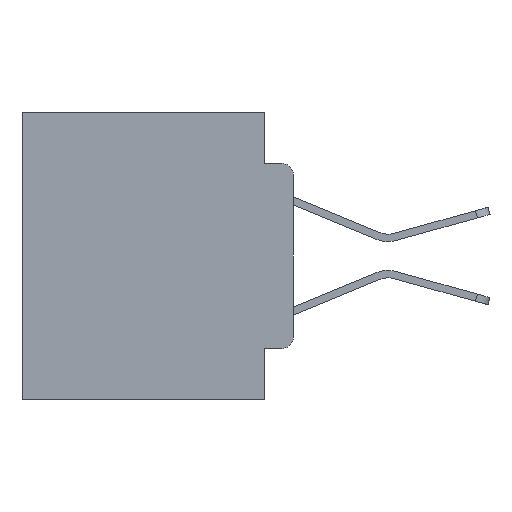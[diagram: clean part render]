
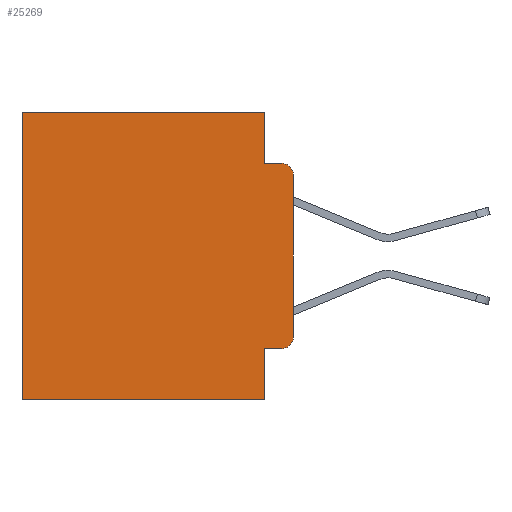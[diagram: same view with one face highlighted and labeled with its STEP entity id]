
A CAD part, left-side view. The second image highlights one B-rep face of the part: STEP entity #25269.
In plain terms, the highlighted planar face has unit normal (-1, 0, 0).
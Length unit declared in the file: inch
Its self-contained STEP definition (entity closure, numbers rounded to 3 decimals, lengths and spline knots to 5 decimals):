
#280 = ORIENTED_EDGE ( 'NONE', *, *, #2390, .T. ) ;
#667 = ORIENTED_EDGE ( 'NONE', *, *, #17414, .T. ) ;
#914 = FACE_OUTER_BOUND ( 'NONE', #7038, .T. ) ;
#1021 = ORIENTED_EDGE ( 'NONE', *, *, #18911, .T. ) ;
#1097 = ORIENTED_EDGE ( 'NONE', *, *, #22683, .F. ) ;
#1190 = CARTESIAN_POINT ( 'NONE',  ( 0.298, 0.051, -0.0885 ) ) ;
#1203 = DIRECTION ( 'NONE',  ( 0., 0., -1. ) ) ;
#1210 = EDGE_CURVE ( 'NONE', #7250, #12770, #22981, .T. ) ;
#1242 = ORIENTED_EDGE ( 'NONE', *, *, #22350, .F. ) ;
#1360 = LINE ( 'NONE', #16604, #23978 ) ;
#1700 = ORIENTED_EDGE ( 'NONE', *, *, #28054, .T. ) ;
#1843 = ORIENTED_EDGE ( 'NONE', *, *, #1210, .F. ) ;
#1898 = ORIENTED_EDGE ( 'NONE', *, *, #25222, .F. ) ;
#2041 = ORIENTED_EDGE ( 'NONE', *, *, #22127, .T. ) ;
#2135 = LINE ( 'NONE', #11034, #7387 ) ;
#2136 = ORIENTED_EDGE ( 'NONE', *, *, #23571, .F. ) ;
#2301 = CARTESIAN_POINT ( 'NONE',  ( 0.298, 0.051, -0.0885 ) ) ;
#2390 = EDGE_CURVE ( 'NONE', #7785, #23870, #25370, .T. ) ;
#3108 = LINE ( 'NONE', #10858, #14094 ) ;
#3114 = LINE ( 'NONE', #22416, #19875 ) ;
#3369 = CARTESIAN_POINT ( 'NONE',  ( 0.298, 0.051, 0. ) ) ;
#4490 = VERTEX_POINT ( 'NONE', #23769 ) ;
#4699 = CIRCLE ( 'NONE', #20246, 0.02 ) ;
#4994 = CARTESIAN_POINT ( 'NONE',  ( 0.298, 0., 0. ) ) ;
#5281 = DIRECTION ( 'NONE',  ( 0., -1., 0. ) ) ;
#5590 = DIRECTION ( 'NONE',  ( 0., 0., -1. ) ) ;
#6176 = LINE ( 'NONE', #26928, #27866 ) ;
#6746 = DIRECTION ( 'NONE',  ( 1., 0., 0. ) ) ;
#6944 = VERTEX_POINT ( 'NONE', #25414 ) ;
#7038 = EDGE_LOOP ( 'NONE', ( #2136, #2041, #1843, #1898, #280, #1700, #1097, #1242, #667, #1021 ) ) ;
#7060 = CARTESIAN_POINT ( 'NONE',  ( 0.298, 0.02, -0.1085 ) ) ;
#7250 = VERTEX_POINT ( 'NONE', #2301 ) ;
#7387 = VECTOR ( 'NONE', #26183, 39.37008 ) ;
#7785 = VERTEX_POINT ( 'NONE', #25985 ) ;
#8514 = CARTESIAN_POINT ( 'NONE',  ( 0.298, 0.473, -0.5 ) ) ;
#8742 = VECTOR ( 'NONE', #20386, 39.37008 ) ;
#9267 = DIRECTION ( 'NONE',  ( 0., 0., -1. ) ) ;
#9916 = AXIS2_PLACEMENT_3D ( 'NONE', #7060, #22276, #9267 ) ;
#10858 = CARTESIAN_POINT ( 'NONE',  ( 0.298, 0.051, 0. ) ) ;
#11034 = CARTESIAN_POINT ( 'NONE',  ( 0.298, 0., -0.5 ) ) ;
#11068 = DIRECTION ( 'NONE',  ( 0., -1., 0. ) ) ;
#12770 = VERTEX_POINT ( 'NONE', #22942 ) ;
#12849 = CARTESIAN_POINT ( 'NONE',  ( 0.298, 0.02, -0.3915 ) ) ;
#14094 = VECTOR ( 'NONE', #23853, 39.37008 ) ;
#15027 = DIRECTION ( 'NONE',  ( 0., 0., -1. ) ) ;
#15436 = CARTESIAN_POINT ( 'NONE',  ( 0.298, 0., -0.1085 ) ) ;
#16604 = CARTESIAN_POINT ( 'NONE',  ( 0.298, 0., 0. ) ) ;
#17414 = EDGE_CURVE ( 'NONE', #6944, #17508, #6176, .T. ) ;
#17508 = VERTEX_POINT ( 'NONE', #25233 ) ;
#18857 = AXIS2_PLACEMENT_3D ( 'NONE', #19806, #6746, #21970 ) ;
#18911 = EDGE_CURVE ( 'NONE', #17508, #24574, #4699, .T. ) ;
#19805 = CARTESIAN_POINT ( 'NONE',  ( 0.298, 0., -0.3915 ) ) ;
#19806 = CARTESIAN_POINT ( 'NONE',  ( 0.298, 0., 0. ) ) ;
#19875 = VECTOR ( 'NONE', #20339, 39.37008 ) ;
#20246 = AXIS2_PLACEMENT_3D ( 'NONE', #12849, #27942, #15027 ) ;
#20339 = DIRECTION ( 'NONE',  ( 0., 0., -1. ) ) ;
#20386 = DIRECTION ( 'NONE',  ( 0., 1., 0. ) ) ;
#21970 = DIRECTION ( 'NONE',  ( 0., 0., -1. ) ) ;
#22127 = EDGE_CURVE ( 'NONE', #23889, #12770, #23058, .T. ) ;
#22276 = DIRECTION ( 'NONE',  ( -1., 0., 0. ) ) ;
#22350 = EDGE_CURVE ( 'NONE', #6944, #4490, #27713, .T. ) ;
#22416 = CARTESIAN_POINT ( 'NONE',  ( 0.298, 0.473, 0. ) ) ;
#22683 = EDGE_CURVE ( 'NONE', #4490, #23783, #2135, .T. ) ;
#22942 = CARTESIAN_POINT ( 'NONE',  ( 0.298, 0.02, -0.0885 ) ) ;
#22981 = LINE ( 'NONE', #1190, #27328 ) ;
#23058 = CIRCLE ( 'NONE', #9916, 0.02 ) ;
#23571 = EDGE_CURVE ( 'NONE', #23889, #24574, #1360, .T. ) ;
#23769 = CARTESIAN_POINT ( 'NONE',  ( 0.298, 0.051, -0.5 ) ) ;
#23783 = VERTEX_POINT ( 'NONE', #8514 ) ;
#23853 = DIRECTION ( 'NONE',  ( 0., 0., -1. ) ) ;
#23870 = VERTEX_POINT ( 'NONE', #27781 ) ;
#23889 = VERTEX_POINT ( 'NONE', #15436 ) ;
#23978 = VECTOR ( 'NONE', #1203, 39.37008 ) ;
#24574 = VERTEX_POINT ( 'NONE', #19805 ) ;
#25222 = EDGE_CURVE ( 'NONE', #7785, #7250, #3108, .T. ) ;
#25233 = CARTESIAN_POINT ( 'NONE',  ( 0.298, 0.02, -0.4115 ) ) ;
#25269 = ADVANCED_FACE ( 'NONE', ( #914 ), #26188, .F. ) ;
#25370 = LINE ( 'NONE', #4994, #8742 ) ;
#25414 = CARTESIAN_POINT ( 'NONE',  ( 0.298, 0.051, -0.4115 ) ) ;
#25985 = CARTESIAN_POINT ( 'NONE',  ( 0.298, 0.051, 0. ) ) ;
#26183 = DIRECTION ( 'NONE',  ( 0., 1., 0. ) ) ;
#26188 = PLANE ( 'NONE',  #18857 ) ;
#26928 = CARTESIAN_POINT ( 'NONE',  ( 0.298, 0.051, -0.4115 ) ) ;
#27068 = VECTOR ( 'NONE', #5590, 39.37008 ) ;
#27328 = VECTOR ( 'NONE', #11068, 39.37008 ) ;
#27713 = LINE ( 'NONE', #3369, #27068 ) ;
#27781 = CARTESIAN_POINT ( 'NONE',  ( 0.298, 0.473, 0. ) ) ;
#27866 = VECTOR ( 'NONE', #5281, 39.37008 ) ;
#27942 = DIRECTION ( 'NONE',  ( -1., 0., 0. ) ) ;
#28054 = EDGE_CURVE ( 'NONE', #23870, #23783, #3114, .T. ) ;
